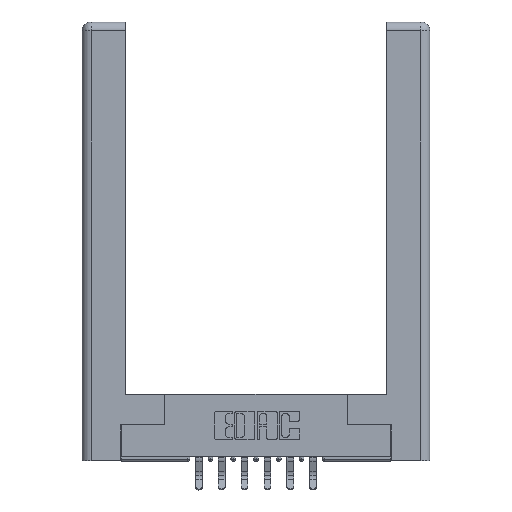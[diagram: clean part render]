
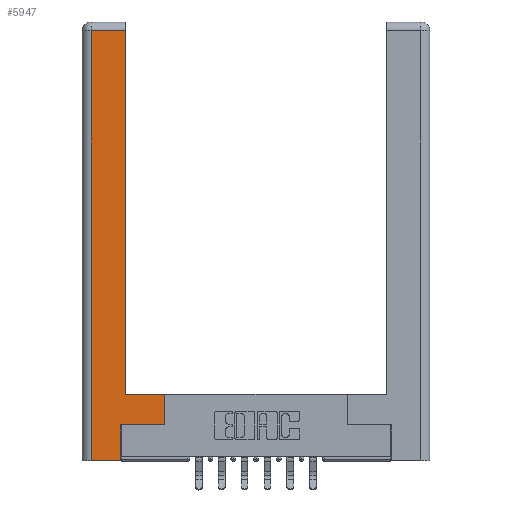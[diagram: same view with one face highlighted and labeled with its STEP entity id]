
A CAD part, top view. The second image highlights one B-rep face of the part: STEP entity #5947.
In plain terms, the highlighted planar face has unit normal (0, 0, 1).
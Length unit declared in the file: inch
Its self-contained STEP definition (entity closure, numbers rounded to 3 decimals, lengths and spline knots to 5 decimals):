
#170 = LINE ( 'NONE', #7879, #9179 ) ;
#372 = VERTEX_POINT ( 'NONE', #9273 ) ;
#459 = VECTOR ( 'NONE', #2563, 39.37008 ) ;
#655 = EDGE_CURVE ( 'NONE', #9267, #7644, #4956, .T. ) ;
#742 = LINE ( 'NONE', #1521, #12324 ) ;
#1290 = LINE ( 'NONE', #2088, #9099 ) ;
#1399 = CARTESIAN_POINT ( 'NONE',  ( 0.0615, 2.94, 0. ) ) ;
#1521 = CARTESIAN_POINT ( 'NONE',  ( 0.565, 0.45, 0. ) ) ;
#1921 = DIRECTION ( 'NONE',  ( 0., 1., 0. ) ) ;
#2088 = CARTESIAN_POINT ( 'NONE',  ( 0.0615, 0., 0. ) ) ;
#2410 = ORIENTED_EDGE ( 'NONE', *, *, #3195, .T. ) ;
#2563 = DIRECTION ( 'NONE',  ( 1., 0., 0. ) ) ;
#2817 = DIRECTION ( 'NONE',  ( -1., 0., 0. ) ) ;
#2878 = CARTESIAN_POINT ( 'NONE',  ( 0.565, 0.245, 0. ) ) ;
#3093 = VERTEX_POINT ( 'NONE', #12481 ) ;
#3104 = CARTESIAN_POINT ( 'NONE',  ( 0.265, 0.245, 0. ) ) ;
#3195 = EDGE_CURVE ( 'NONE', #8734, #3093, #742, .T. ) ;
#3366 = CARTESIAN_POINT ( 'NONE',  ( 0.0615, 2.94, 0. ) ) ;
#3802 = DIRECTION ( 'NONE',  ( 1., 0., 0. ) ) ;
#4095 = DIRECTION ( 'NONE',  ( 0., -1., 0. ) ) ;
#4119 = EDGE_CURVE ( 'NONE', #12215, #10569, #12639, .T. ) ;
#4338 = ORIENTED_EDGE ( 'NONE', *, *, #13658, .T. ) ;
#4956 = LINE ( 'NONE', #1399, #11591 ) ;
#5208 = EDGE_CURVE ( 'NONE', #3093, #8615, #170, .T. ) ;
#5459 = CARTESIAN_POINT ( 'NONE',  ( 0.265, 0., 0. ) ) ;
#5947 = ADVANCED_FACE ( 'NONE', ( #10552 ), #9223, .F. ) ;
#5974 = CARTESIAN_POINT ( 'NONE',  ( 0., 0., 0. ) ) ;
#6077 = CARTESIAN_POINT ( 'NONE',  ( 0.0615, 0., 0. ) ) ;
#7074 = LINE ( 'NONE', #11253, #8074 ) ;
#7123 = ORIENTED_EDGE ( 'NONE', *, *, #4119, .T. ) ;
#7644 = VERTEX_POINT ( 'NONE', #3366 ) ;
#7802 = EDGE_LOOP ( 'NONE', ( #4338, #12815, #9521, #7123, #9155, #8621, #2410, #12116 ) ) ;
#7874 = DIRECTION ( 'NONE',  ( -1., 0., 0. ) ) ;
#7879 = CARTESIAN_POINT ( 'NONE',  ( 0.295, 0.45, 0. ) ) ;
#8074 = VECTOR ( 'NONE', #11306, 39.37008 ) ;
#8615 = VERTEX_POINT ( 'NONE', #8681 ) ;
#8621 = ORIENTED_EDGE ( 'NONE', *, *, #13085, .T. ) ;
#8681 = CARTESIAN_POINT ( 'NONE',  ( 0.295, 0.45, 0. ) ) ;
#8734 = VERTEX_POINT ( 'NONE', #2878 ) ;
#9031 = AXIS2_PLACEMENT_3D ( 'NONE', #5974, #13430, #11356 ) ;
#9099 = VECTOR ( 'NONE', #4095, 39.37008 ) ;
#9155 = ORIENTED_EDGE ( 'NONE', *, *, #11943, .T. ) ;
#9179 = VECTOR ( 'NONE', #2817, 39.37008 ) ;
#9223 = PLANE ( 'NONE',  #9031 ) ;
#9267 = VERTEX_POINT ( 'NONE', #12093 ) ;
#9273 = CARTESIAN_POINT ( 'NONE',  ( 0.265, 0.245, 0. ) ) ;
#9521 = ORIENTED_EDGE ( 'NONE', *, *, #11023, .T. ) ;
#9849 = VECTOR ( 'NONE', #3802, 39.37008 ) ;
#10104 = CARTESIAN_POINT ( 'NONE',  ( 0.565, 0.245, 0. ) ) ;
#10157 = CARTESIAN_POINT ( 'NONE',  ( 0.265, 0., 0. ) ) ;
#10552 = FACE_OUTER_BOUND ( 'NONE', #7802, .T. ) ;
#10569 = VERTEX_POINT ( 'NONE', #5459 ) ;
#10878 = VECTOR ( 'NONE', #1921, 39.37008 ) ;
#11023 = EDGE_CURVE ( 'NONE', #7644, #12215, #1290, .T. ) ;
#11130 = DIRECTION ( 'NONE',  ( 0., 1., 0. ) ) ;
#11253 = CARTESIAN_POINT ( 'NONE',  ( 0.295, 3., 0. ) ) ;
#11306 = DIRECTION ( 'NONE',  ( 0., 1., 0. ) ) ;
#11356 = DIRECTION ( 'NONE',  ( -1., 0., 0. ) ) ;
#11591 = VECTOR ( 'NONE', #7874, 39.37008 ) ;
#11943 = EDGE_CURVE ( 'NONE', #10569, #372, #13709, .T. ) ;
#12093 = CARTESIAN_POINT ( 'NONE',  ( 0.295, 2.94, 0. ) ) ;
#12116 = ORIENTED_EDGE ( 'NONE', *, *, #5208, .T. ) ;
#12215 = VERTEX_POINT ( 'NONE', #6077 ) ;
#12324 = VECTOR ( 'NONE', #11130, 39.37008 ) ;
#12481 = CARTESIAN_POINT ( 'NONE',  ( 0.565, 0.45, 0. ) ) ;
#12639 = LINE ( 'NONE', #10157, #9849 ) ;
#12815 = ORIENTED_EDGE ( 'NONE', *, *, #655, .T. ) ;
#13085 = EDGE_CURVE ( 'NONE', #372, #8734, #13578, .T. ) ;
#13430 = DIRECTION ( 'NONE',  ( 0., 0., -1. ) ) ;
#13578 = LINE ( 'NONE', #10104, #459 ) ;
#13658 = EDGE_CURVE ( 'NONE', #8615, #9267, #7074, .T. ) ;
#13709 = LINE ( 'NONE', #3104, #10878 ) ;
